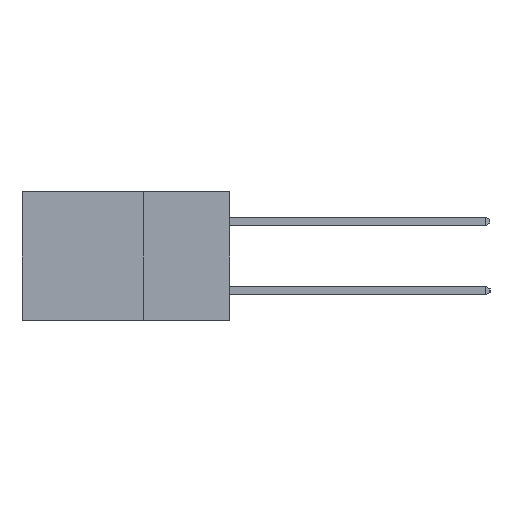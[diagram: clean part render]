
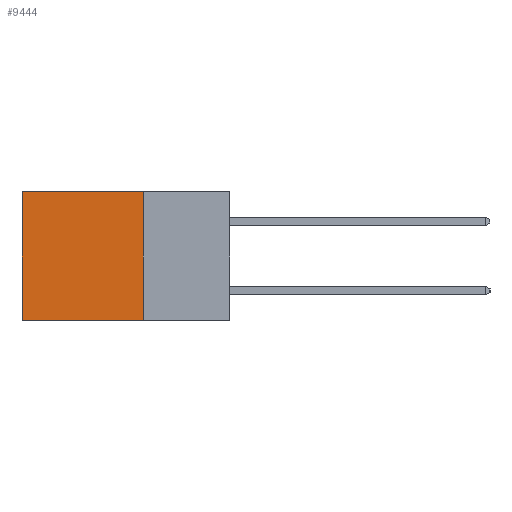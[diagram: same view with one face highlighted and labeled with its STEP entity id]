
A CAD part, left-side view. The second image highlights one B-rep face of the part: STEP entity #9444.
In plain terms, the highlighted planar face has unit normal (-1, 0, 0).
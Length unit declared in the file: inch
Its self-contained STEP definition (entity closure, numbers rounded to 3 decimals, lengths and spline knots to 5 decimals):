
#163 = VECTOR ( 'NONE', #2811, 39.37008 ) ;
#171 = VECTOR ( 'NONE', #8907, 39.37008 ) ;
#1248 = CARTESIAN_POINT ( 'NONE',  ( 0.2615, 0.25, -0.37 ) ) ;
#1489 = DIRECTION ( 'NONE',  ( 0., 0., -1. ) ) ;
#1709 = ORIENTED_EDGE ( 'NONE', *, *, #20227, .T. ) ;
#2811 = DIRECTION ( 'NONE',  ( 0., 1., 0. ) ) ;
#3102 = EDGE_CURVE ( 'NONE', #23707, #9382, #10714, .T. ) ;
#3388 = EDGE_LOOP ( 'NONE', ( #5215, #20530, #23675, #1709 ) ) ;
#4060 = AXIS2_PLACEMENT_3D ( 'NONE', #11343, #13274, #1489 ) ;
#4584 = VERTEX_POINT ( 'NONE', #6230 ) ;
#5072 = CARTESIAN_POINT ( 'NONE',  ( 0.2615, 0.6, -0.37 ) ) ;
#5193 = CARTESIAN_POINT ( 'NONE',  ( 0.2615, 0.25, 0. ) ) ;
#5215 = ORIENTED_EDGE ( 'NONE', *, *, #11228, .T. ) ;
#6230 = CARTESIAN_POINT ( 'NONE',  ( 0.2615, 0.6, 0. ) ) ;
#7137 = LINE ( 'NONE', #23986, #16812 ) ;
#8340 = FACE_OUTER_BOUND ( 'NONE', #3388, .T. ) ;
#8907 = DIRECTION ( 'NONE',  ( 0., 0., -1. ) ) ;
#9089 = DIRECTION ( 'NONE',  ( 0., 1., 0. ) ) ;
#9382 = VERTEX_POINT ( 'NONE', #1248 ) ;
#9444 = ADVANCED_FACE ( 'NONE', ( #8340 ), #22730, .F. ) ;
#10706 = LINE ( 'NONE', #12623, #163 ) ;
#10714 = LINE ( 'NONE', #19694, #171 ) ;
#11045 = LINE ( 'NONE', #5193, #15585 ) ;
#11228 = EDGE_CURVE ( 'NONE', #4584, #12004, #7137, .T. ) ;
#11343 = CARTESIAN_POINT ( 'NONE',  ( 0.2615, 0.25, -0.37 ) ) ;
#12004 = VERTEX_POINT ( 'NONE', #5072 ) ;
#12623 = CARTESIAN_POINT ( 'NONE',  ( 0.2615, 0.25, -0.37 ) ) ;
#12642 = DIRECTION ( 'NONE',  ( 0., 0., -1. ) ) ;
#13274 = DIRECTION ( 'NONE',  ( 1., 0., 0. ) ) ;
#14018 = EDGE_CURVE ( 'NONE', #9382, #12004, #10706, .T. ) ;
#15585 = VECTOR ( 'NONE', #9089, 39.37008 ) ;
#16812 = VECTOR ( 'NONE', #12642, 39.37008 ) ;
#19694 = CARTESIAN_POINT ( 'NONE',  ( 0.2615, 0.25, -0.37 ) ) ;
#20227 = EDGE_CURVE ( 'NONE', #23707, #4584, #11045, .T. ) ;
#20530 = ORIENTED_EDGE ( 'NONE', *, *, #14018, .F. ) ;
#22730 = PLANE ( 'NONE',  #4060 ) ;
#23675 = ORIENTED_EDGE ( 'NONE', *, *, #3102, .F. ) ;
#23707 = VERTEX_POINT ( 'NONE', #24777 ) ;
#23986 = CARTESIAN_POINT ( 'NONE',  ( 0.2615, 0.6, -0.37 ) ) ;
#24777 = CARTESIAN_POINT ( 'NONE',  ( 0.2615, 0.25, 0. ) ) ;
